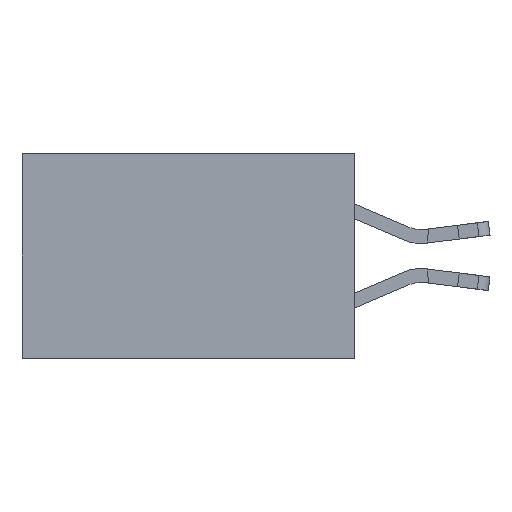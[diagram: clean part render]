
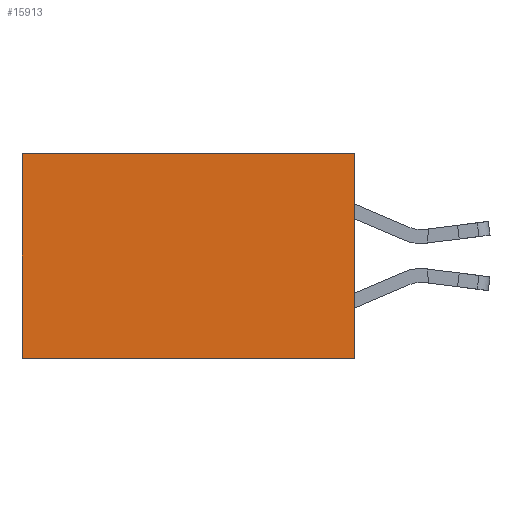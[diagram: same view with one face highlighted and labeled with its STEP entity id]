
A CAD part, left-side view. The second image highlights one B-rep face of the part: STEP entity #15913.
In plain terms, the highlighted planar face has unit normal (-1, 0, 0).
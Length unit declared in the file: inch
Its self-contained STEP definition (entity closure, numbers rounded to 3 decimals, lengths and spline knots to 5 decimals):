
#75 = ORIENTED_EDGE ( 'NONE', *, *, #16028, .F. ) ;
#150 = DIRECTION ( 'NONE',  ( 1., 0., 0. ) ) ;
#973 = EDGE_CURVE ( 'NONE', #18305, #8527, #13194, .T. ) ;
#2248 = FACE_OUTER_BOUND ( 'NONE', #12438, .T. ) ;
#2907 = CARTESIAN_POINT ( 'NONE',  ( 0.298, 0., 0. ) ) ;
#2978 = DIRECTION ( 'NONE',  ( 0., 1., 0. ) ) ;
#3109 = VECTOR ( 'NONE', #16127, 39.37008 ) ;
#3843 = LINE ( 'NONE', #13269, #11394 ) ;
#4281 = EDGE_CURVE ( 'NONE', #8527, #15256, #6517, .T. ) ;
#4395 = AXIS2_PLACEMENT_3D ( 'NONE', #8781, #150, #10176 ) ;
#4767 = DIRECTION ( 'NONE',  ( 0., 0., -1. ) ) ;
#5580 = ORIENTED_EDGE ( 'NONE', *, *, #973, .T. ) ;
#6062 = ORIENTED_EDGE ( 'NONE', *, *, #4281, .T. ) ;
#6295 = CARTESIAN_POINT ( 'NONE',  ( 0.298, 0., -0.37 ) ) ;
#6517 = LINE ( 'NONE', #8039, #17260 ) ;
#8039 = CARTESIAN_POINT ( 'NONE',  ( 0.298, 0.6, 0. ) ) ;
#8263 = CARTESIAN_POINT ( 'NONE',  ( 0.298, 0.6, -0.37 ) ) ;
#8502 = DIRECTION ( 'NONE',  ( 0., 0., -1. ) ) ;
#8527 = VERTEX_POINT ( 'NONE', #9990 ) ;
#8781 = CARTESIAN_POINT ( 'NONE',  ( 0.298, 0., 0. ) ) ;
#9990 = CARTESIAN_POINT ( 'NONE',  ( 0.298, 0.6, 0. ) ) ;
#10112 = PLANE ( 'NONE',  #4395 ) ;
#10176 = DIRECTION ( 'NONE',  ( 0., 0., -1. ) ) ;
#11394 = VECTOR ( 'NONE', #4767, 39.37008 ) ;
#11714 = CARTESIAN_POINT ( 'NONE',  ( 0.298, 0., -0.37 ) ) ;
#12438 = EDGE_LOOP ( 'NONE', ( #6062, #16324, #75, #5580 ) ) ;
#13194 = LINE ( 'NONE', #2907, #13644 ) ;
#13269 = CARTESIAN_POINT ( 'NONE',  ( 0.298, 0., 0. ) ) ;
#13644 = VECTOR ( 'NONE', #2978, 39.37008 ) ;
#13883 = CARTESIAN_POINT ( 'NONE',  ( 0.298, 0., 0. ) ) ;
#15256 = VERTEX_POINT ( 'NONE', #8263 ) ;
#15913 = ADVANCED_FACE ( 'NONE', ( #2248 ), #10112, .F. ) ;
#16028 = EDGE_CURVE ( 'NONE', #18305, #17929, #3843, .T. ) ;
#16127 = DIRECTION ( 'NONE',  ( 0., 1., 0. ) ) ;
#16324 = ORIENTED_EDGE ( 'NONE', *, *, #16777, .F. ) ;
#16777 = EDGE_CURVE ( 'NONE', #17929, #15256, #17775, .T. ) ;
#17260 = VECTOR ( 'NONE', #8502, 39.37008 ) ;
#17775 = LINE ( 'NONE', #6295, #3109 ) ;
#17929 = VERTEX_POINT ( 'NONE', #11714 ) ;
#18305 = VERTEX_POINT ( 'NONE', #13883 ) ;
